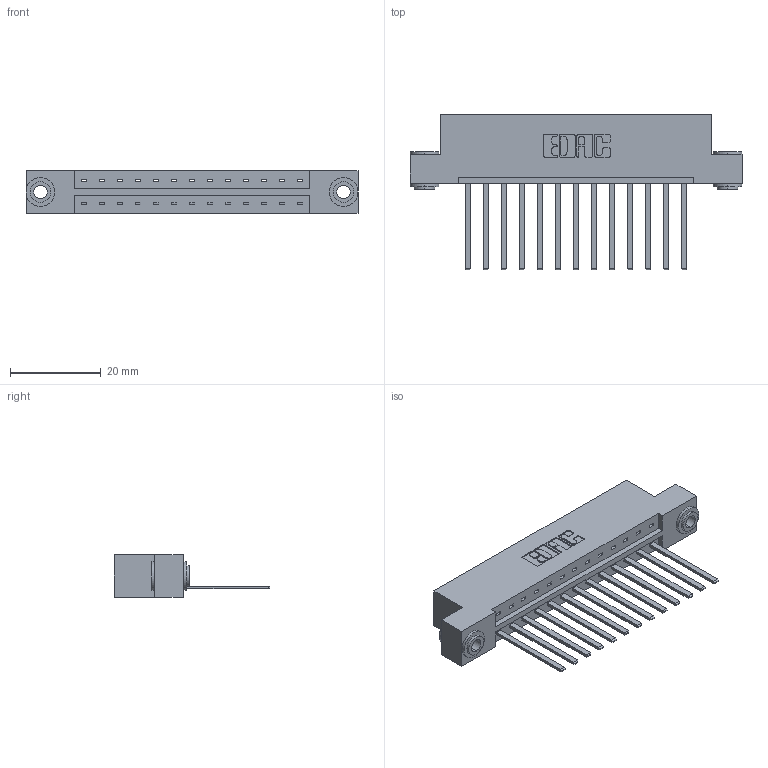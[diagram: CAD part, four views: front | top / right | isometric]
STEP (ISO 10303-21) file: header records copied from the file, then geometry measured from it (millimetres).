
FILE_DESCRIPTION (( 'STEP AP203' ), '1' );
FILE_NAME ('833-013-544-103.STEP', '2020-05-31T00:20:27', ( '' ), ( '' ), 'SwSTEP 2.0', 'SolidWorks 2020', '' );
FILE_SCHEMA (( 'CONFIG_CONTROL_DESIGN' ));
Length unit declared in the file: inch
Products named in the file (4): 345-292-001_345-293-144; 833 Part_Flush - .156 Dia - TH; 345-250-002_345-250-002-102; 833-013-544-103
Assembly tree (16 placements, depth 2):
  833-013-544-103
    833 Part_Flush - .156 Dia - TH
    345-292-001_345-293-144  x13
    345-250-002_345-250-002-102  x2
Bounding box: 73.05 x 34.3 x 9.4 mm (x, y, z)
Volume: 7271.5 mm3; surface area: 8394.9 mm2
Topology: 16 solids, 16 shells, 828 faces, 2441 edges, 1606 vertices
Faces by surface type: plane 574, cylinder 246, cone 8
Entity records: 12164 total; most frequent: CARTESIAN_POINT 2080, ORIENTED_EDGE 2022, DIRECTION 1843, EDGE_CURVE 1011, VECTOR 863, LINE 863, VERTEX_POINT 670, AXIS2_PLACEMENT_3D 490
